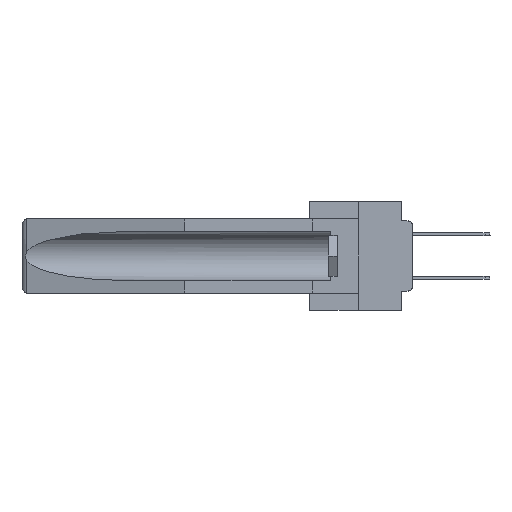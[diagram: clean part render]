
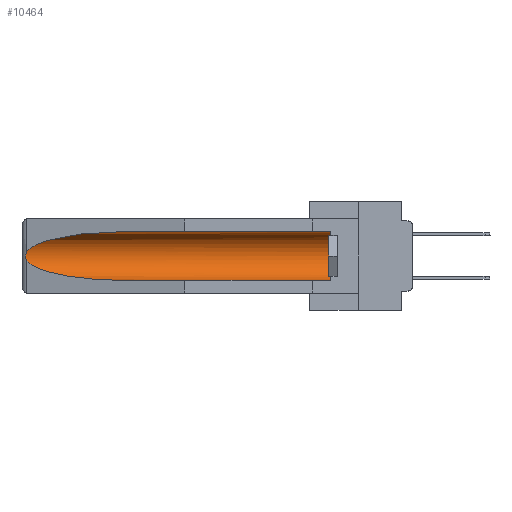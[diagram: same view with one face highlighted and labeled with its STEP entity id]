
A CAD part, left-side view. The second image highlights one B-rep face of the part: STEP entity #10464.
In plain terms, the highlighted cylindrical face has radius 2.857 mm (diameter 5.715 mm), a partial arc.
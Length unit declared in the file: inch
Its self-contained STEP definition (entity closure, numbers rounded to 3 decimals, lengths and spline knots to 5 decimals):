
#320 = CARTESIAN_POINT ( 'NONE',  ( 0.25451, 1.48313, -0.24835 ) ) ;
#528 = CARTESIAN_POINT ( 'NONE',  ( 0.26537, 1.52718, -0.14972 ) ) ;
#593 = CARTESIAN_POINT ( 'NONE',  ( 0.155, 0.126, -0.1715 ) ) ;
#1795 = CARTESIAN_POINT ( 'NONE',  ( 0.26537, 1.52718, -0.14972 ) ) ;
#3219 = CARTESIAN_POINT ( 'NONE',  ( 0.2675, 1.53308, -0.17534 ) ) ;
#3461 = DIRECTION ( 'NONE',  ( 0., -1., 0. ) ) ;
#5839 = CARTESIAN_POINT ( 'NONE',  ( 0.26537, 1.52718, -0.19328 ) ) ;
#6075 = DIRECTION ( 'NONE',  ( 0., 0., 1. ) ) ;
#6412 = CARTESIAN_POINT ( 'NONE',  ( 0.26597, 1.52961, -0.15275 ) ) ;
#6831 = VERTEX_POINT ( 'NONE', #16558 ) ;
#7461 = LINE ( 'NONE', #28976, #10603 ) ;
#7795 = CARTESIAN_POINT ( 'NONE',  ( 0.155, 1.07973, -0.284 ) ) ;
#8946 = CARTESIAN_POINT ( 'NONE',  ( 0.26537, 1.52718, -0.14972 ) ) ;
#9111 = CARTESIAN_POINT ( 'NONE',  ( 0.21114, 1.30732, -0.059 ) ) ;
#9473 = VERTEX_POINT ( 'NONE', #29323 ) ;
#9496 = AXIS2_PLACEMENT_3D ( 'NONE', #593, #3461, #11682 ) ;
#9797 = DIRECTION ( 'NONE',  ( 0., 1., 0. ) ) ;
#10464 = ADVANCED_FACE ( 'NONE', ( #19606 ), #22460, .F. ) ;
#10603 = VECTOR ( 'NONE', #9797, 39.37008 ) ;
#11079 = CARTESIAN_POINT ( 'NONE',  ( 0.25451, 1.48313, -0.09465 ) ) ;
#11273 = CARTESIAN_POINT ( 'NONE',  ( 0.155, -0.30754, -0.1715 ) ) ;
#11279 = ORIENTED_EDGE ( 'NONE', *, *, #16876, .T. ) ;
#11296 = EDGE_CURVE ( 'NONE', #19813, #6831, #15105, .T. ) ;
#11682 = DIRECTION ( 'NONE',  ( 0., 0., 1. ) ) ;
#12171 = LINE ( 'NONE', #28136, #14929 ) ;
#12471 = ORIENTED_EDGE ( 'NONE', *, *, #32768, .F. ) ;
#13592 = ORIENTED_EDGE ( 'NONE', *, *, #20411, .T. ) ;
#13945 = CARTESIAN_POINT ( 'NONE',  ( 0.26655, 1.53094, -0.18657 ) ) ;
#14237 = CARTESIAN_POINT ( 'NONE',  ( 0.155, 1.07973, -0.284 ) ) ;
#14929 = VECTOR ( 'NONE', #30649, 39.37008 ) ;
#15105 = CIRCLE ( 'NONE', #9496, 0.1125 ) ;
#16558 = CARTESIAN_POINT ( 'NONE',  ( 0.155, 0.126, -0.059 ) ) ;
#16876 = EDGE_CURVE ( 'NONE', #6831, #9473, #12171, .T. ) ;
#16978 = B_SPLINE_CURVE_WITH_KNOTS ( 'NONE', 3,
 ( #8946, #6412, #22609, #25447, #17099, #3219, #27427, #13945, #24750, #17269 ),
 .UNSPECIFIED., .F., .F.,
 ( 4, 2, 2, 2, 4 ),
 ( 0., 0.00029, 0.00058, 0.00087, 0.00117 ),
 .UNSPECIFIED. ) ;
#17099 = CARTESIAN_POINT ( 'NONE',  ( 0.2675, 1.53308, -0.16763 ) ) ;
#17269 = CARTESIAN_POINT ( 'NONE',  ( 0.26537, 1.52718, -0.19328 ) ) ;
#18047 = ORIENTED_EDGE ( 'NONE', *, *, #24301, .T. ) ;
#19049 = ORIENTED_EDGE ( 'NONE', *, *, #11296, .T. ) ;
#19371 = VERTEX_POINT ( 'NONE', #7795 ) ;
#19606 = FACE_OUTER_BOUND ( 'NONE', #21488, .T. ) ;
#19813 = VERTEX_POINT ( 'NONE', #26756 ) ;
#20351 = EDGE_CURVE ( 'NONE', #9473, #27311, #34871, .T. ) ;
#20411 = EDGE_CURVE ( 'NONE', #27311, #34273, #16978, .T. ) ;
#21461 =( BOUNDED_CURVE ( )  B_SPLINE_CURVE ( 3, ( #5839, #320, #30756, #14237 ),
 .UNSPECIFIED., .F., .F. ) 
 B_SPLINE_CURVE_WITH_KNOTS ( ( 4, 4 ),
 ( 0.1948, 1.5708 ),
 .UNSPECIFIED. ) 
 CURVE ( )  GEOMETRIC_REPRESENTATION_ITEM ( )  RATIONAL_B_SPLINE_CURVE ( ( 1., 0.848, 0.848, 1. ) ) 
 REPRESENTATION_ITEM ( '' )  );
#21488 = EDGE_LOOP ( 'NONE', ( #33133, #13592, #18047, #12471, #19049, #11279 ) ) ;
#22460 = CYLINDRICAL_SURFACE ( 'NONE', #25138, 0.1125 ) ;
#22609 = CARTESIAN_POINT ( 'NONE',  ( 0.26654, 1.53092, -0.15636 ) ) ;
#24301 = EDGE_CURVE ( 'NONE', #34273, #19371, #21461, .T. ) ;
#24750 = CARTESIAN_POINT ( 'NONE',  ( 0.26597, 1.5296, -0.19026 ) ) ;
#25138 = AXIS2_PLACEMENT_3D ( 'NONE', #11273, #30469, #6075 ) ;
#25447 = CARTESIAN_POINT ( 'NONE',  ( 0.2673, 1.5327, -0.16383 ) ) ;
#26756 = CARTESIAN_POINT ( 'NONE',  ( 0.155, 0.126, -0.284 ) ) ;
#27311 = VERTEX_POINT ( 'NONE', #1795 ) ;
#27427 = CARTESIAN_POINT ( 'NONE',  ( 0.2673, 1.53269, -0.17917 ) ) ;
#27785 = CARTESIAN_POINT ( 'NONE',  ( 0.26537, 1.52718, -0.19328 ) ) ;
#28136 = CARTESIAN_POINT ( 'NONE',  ( 0.155, -0.30754, -0.059 ) ) ;
#28976 = CARTESIAN_POINT ( 'NONE',  ( 0.155, -0.30754, -0.284 ) ) ;
#29323 = CARTESIAN_POINT ( 'NONE',  ( 0.155, 1.07973, -0.059 ) ) ;
#30469 = DIRECTION ( 'NONE',  ( 0., 1., 0. ) ) ;
#30649 = DIRECTION ( 'NONE',  ( 0., 1., 0. ) ) ;
#30756 = CARTESIAN_POINT ( 'NONE',  ( 0.21114, 1.30732, -0.284 ) ) ;
#32241 = CARTESIAN_POINT ( 'NONE',  ( 0.155, 1.07973, -0.059 ) ) ;
#32768 = EDGE_CURVE ( 'NONE', #19813, #19371, #7461, .T. ) ;
#33133 = ORIENTED_EDGE ( 'NONE', *, *, #20351, .T. ) ;
#34273 = VERTEX_POINT ( 'NONE', #27785 ) ;
#34871 =( BOUNDED_CURVE ( )  B_SPLINE_CURVE ( 3, ( #32241, #9111, #11079, #528 ),
 .UNSPECIFIED., .F., .F. ) 
 B_SPLINE_CURVE_WITH_KNOTS ( ( 4, 4 ),
 ( 4.71239, 6.08839 ),
 .UNSPECIFIED. ) 
 CURVE ( )  GEOMETRIC_REPRESENTATION_ITEM ( )  RATIONAL_B_SPLINE_CURVE ( ( 1., 0.848, 0.848, 1. ) ) 
 REPRESENTATION_ITEM ( '' )  );
